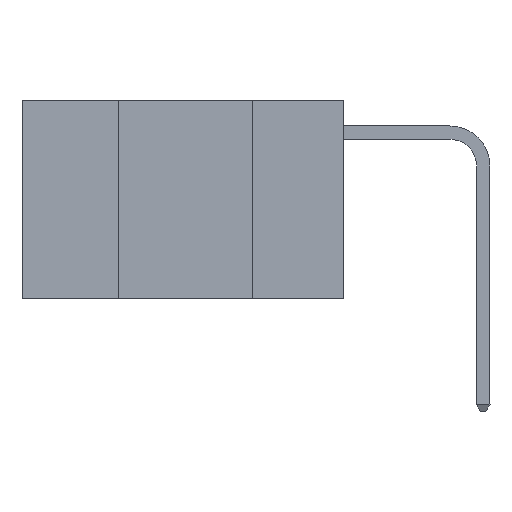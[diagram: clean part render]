
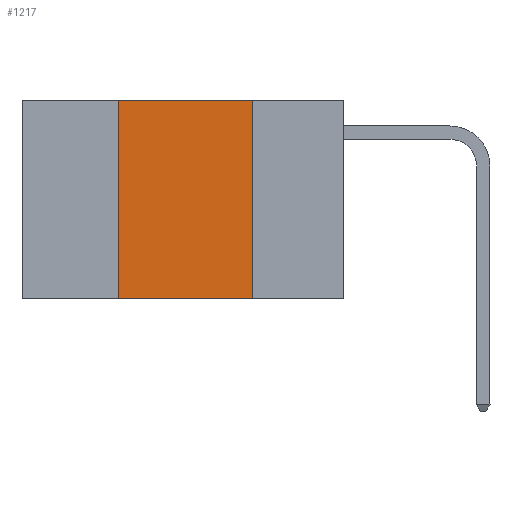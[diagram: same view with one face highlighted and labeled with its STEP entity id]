
A CAD part, left-side view. The second image highlights one B-rep face of the part: STEP entity #1217.
In plain terms, the highlighted planar face has unit normal (-1, 0, 0).
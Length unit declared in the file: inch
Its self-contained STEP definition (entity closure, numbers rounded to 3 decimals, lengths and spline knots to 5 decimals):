
#408 = DIRECTION ( 'NONE',  ( 0., 0., -1. ) ) ;
#795 = CARTESIAN_POINT ( 'NONE',  ( 0., 0.17, 0. ) ) ;
#934 = DIRECTION ( 'NONE',  ( 0., -1., 0. ) ) ;
#1136 = CARTESIAN_POINT ( 'NONE',  ( 0., 0.6, -0.37 ) ) ;
#1217 = ADVANCED_FACE ( 'NONE', ( #4965 ), #8272, .F. ) ;
#1341 = CARTESIAN_POINT ( 'NONE',  ( 0., 0.17, -0.37 ) ) ;
#1877 = DIRECTION ( 'NONE',  ( 0., 0., -1. ) ) ;
#3029 = VECTOR ( 'NONE', #9993, 39.37008 ) ;
#3319 = LINE ( 'NONE', #9893, #3029 ) ;
#3672 = VECTOR ( 'NONE', #934, 39.37008 ) ;
#3754 = LINE ( 'NONE', #1136, #3672 ) ;
#4184 = EDGE_CURVE ( 'NONE', #6170, #6267, #3319, .T. ) ;
#4631 = LINE ( 'NONE', #5515, #7422 ) ;
#4965 = FACE_OUTER_BOUND ( 'NONE', #5955, .T. ) ;
#5501 = DIRECTION ( 'NONE',  ( 0., -1., 0. ) ) ;
#5515 = CARTESIAN_POINT ( 'NONE',  ( 0., 0.6, 0. ) ) ;
#5629 = VECTOR ( 'NONE', #1877, 39.37008 ) ;
#5705 = EDGE_CURVE ( 'NONE', #6170, #10192, #3754, .T. ) ;
#5955 = EDGE_LOOP ( 'NONE', ( #11020, #7902, #8881, #8709 ) ) ;
#6170 = VERTEX_POINT ( 'NONE', #10291 ) ;
#6267 = VERTEX_POINT ( 'NONE', #6460 ) ;
#6299 = EDGE_CURVE ( 'NONE', #6267, #7440, #4631, .T. ) ;
#6460 = CARTESIAN_POINT ( 'NONE',  ( 0., 0.42, 0. ) ) ;
#6972 = EDGE_CURVE ( 'NONE', #7440, #10192, #8269, .T. ) ;
#7422 = VECTOR ( 'NONE', #5501, 39.37008 ) ;
#7423 = CARTESIAN_POINT ( 'NONE',  ( 0., 0.6, 0. ) ) ;
#7440 = VERTEX_POINT ( 'NONE', #9045 ) ;
#7571 = DIRECTION ( 'NONE',  ( 1., 0., 0. ) ) ;
#7902 = ORIENTED_EDGE ( 'NONE', *, *, #6299, .F. ) ;
#8269 = LINE ( 'NONE', #795, #5629 ) ;
#8272 = PLANE ( 'NONE',  #10592 ) ;
#8709 = ORIENTED_EDGE ( 'NONE', *, *, #5705, .T. ) ;
#8881 = ORIENTED_EDGE ( 'NONE', *, *, #4184, .F. ) ;
#9045 = CARTESIAN_POINT ( 'NONE',  ( 0., 0.17, 0. ) ) ;
#9893 = CARTESIAN_POINT ( 'NONE',  ( 0., 0.42, 0. ) ) ;
#9993 = DIRECTION ( 'NONE',  ( 0., 0., 1. ) ) ;
#10192 = VERTEX_POINT ( 'NONE', #1341 ) ;
#10291 = CARTESIAN_POINT ( 'NONE',  ( 0., 0.42, -0.37 ) ) ;
#10592 = AXIS2_PLACEMENT_3D ( 'NONE', #7423, #7571, #408 ) ;
#11020 = ORIENTED_EDGE ( 'NONE', *, *, #6972, .F. ) ;
